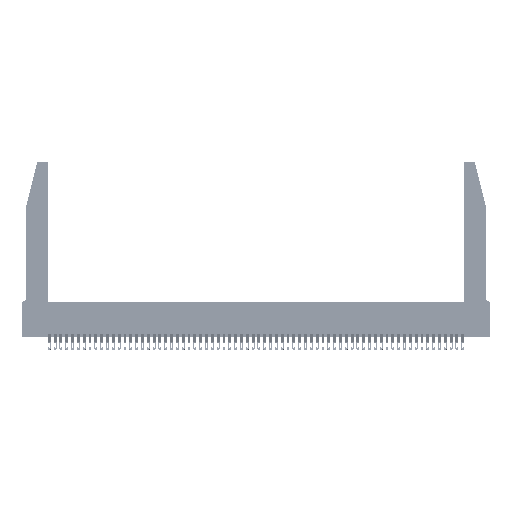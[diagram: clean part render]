
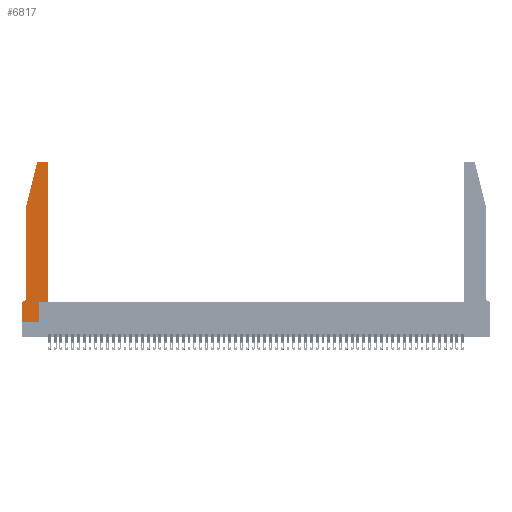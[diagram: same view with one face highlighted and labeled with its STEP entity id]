
A CAD part, top view. The second image highlights one B-rep face of the part: STEP entity #6817.
In plain terms, the highlighted planar face has unit normal (0, 0, 1).
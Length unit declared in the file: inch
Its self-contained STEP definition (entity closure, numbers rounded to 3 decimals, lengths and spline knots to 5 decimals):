
#1048 = VERTEX_POINT ( 'NONE', #35575 ) ;
#1233 = VERTEX_POINT ( 'NONE', #45393 ) ;
#1956 = DIRECTION ( 'NONE',  ( 0., 1., 0. ) ) ;
#2176 = CARTESIAN_POINT ( 'NONE',  ( 0.284, 2.75, 0.37 ) ) ;
#3952 = LINE ( 'NONE', #24320, #27723 ) ;
#5783 = AXIS2_PLACEMENT_3D ( 'NONE', #39515, #8673, #39702 ) ;
#5968 = LINE ( 'NONE', #25566, #29686 ) ;
#6336 = DIRECTION ( 'NONE',  ( 0., 0., 1. ) ) ;
#6624 = DIRECTION ( 'NONE',  ( -0.239, -0.971, 0. ) ) ;
#6817 = ADVANCED_FACE ( 'NONE', ( #33109 ), #57195, .T. ) ;
#8673 = DIRECTION ( 'NONE',  ( 0., 0., 1. ) ) ;
#8991 = LINE ( 'NONE', #37666, #54625 ) ;
#9388 = VECTOR ( 'NONE', #22037, 39.37008 ) ;
#9606 = ORIENTED_EDGE ( 'NONE', *, *, #15689, .T. ) ;
#9902 = VECTOR ( 'NONE', #38142, 39.37008 ) ;
#10875 = CARTESIAN_POINT ( 'NONE',  ( 0.0055, 0.35, 0.37 ) ) ;
#11460 = VERTEX_POINT ( 'NONE', #50817 ) ;
#11614 = CARTESIAN_POINT ( 'NONE',  ( 0.0755, 0.35, 0.37 ) ) ;
#11768 = CARTESIAN_POINT ( 'NONE',  ( 0.2605, 2.75, 0.37 ) ) ;
#12643 = CARTESIAN_POINT ( 'NONE',  ( 0.0755, 2., 0.37 ) ) ;
#13379 = EDGE_CURVE ( 'NONE', #26107, #41893, #55139, .T. ) ;
#13888 = DIRECTION ( 'NONE',  ( 0., 0., -1. ) ) ;
#14454 = DIRECTION ( 'NONE',  ( 1., 0., 0. ) ) ;
#15689 = EDGE_CURVE ( 'NONE', #21227, #52865, #30096, .T. ) ;
#15892 = CARTESIAN_POINT ( 'NONE',  ( 0.4505, 0.35, 0.37 ) ) ;
#17640 = EDGE_CURVE ( 'NONE', #41893, #39931, #25126, .T. ) ;
#17694 = CARTESIAN_POINT ( 'NONE',  ( 0.4505, 2.72, 0.37 ) ) ;
#17924 = ORIENTED_EDGE ( 'NONE', *, *, #28696, .T. ) ;
#19834 = DIRECTION ( 'NONE',  ( 0., -1., 0. ) ) ;
#20935 = ORIENTED_EDGE ( 'NONE', *, *, #45521, .T. ) ;
#21110 = VECTOR ( 'NONE', #42333, 39.37008 ) ;
#21181 = EDGE_LOOP ( 'NONE', ( #31744, #45854, #48638, #26102, #39755, #17924, #37886, #22853, #50915, #9606, #20935, #30724 ) ) ;
#21227 = VERTEX_POINT ( 'NONE', #34133 ) ;
#21753 = VECTOR ( 'NONE', #14454, 39.37008 ) ;
#21771 = EDGE_CURVE ( 'NONE', #11460, #1233, #30501, .T. ) ;
#22037 = DIRECTION ( 'NONE',  ( 0., -1., 0. ) ) ;
#22853 = ORIENTED_EDGE ( 'NONE', *, *, #29841, .T. ) ;
#23035 = VERTEX_POINT ( 'NONE', #49977 ) ;
#24320 = CARTESIAN_POINT ( 'NONE',  ( 0.4505, 0.35, 0.37 ) ) ;
#25126 = LINE ( 'NONE', #11768, #47162 ) ;
#25566 = CARTESIAN_POINT ( 'NONE',  ( 0.2865, 0.35, 0.37 ) ) ;
#26102 = ORIENTED_EDGE ( 'NONE', *, *, #42022, .T. ) ;
#26107 = VERTEX_POINT ( 'NONE', #17694 ) ;
#26424 = DIRECTION ( 'NONE',  ( 0., 0., 1. ) ) ;
#27723 = VECTOR ( 'NONE', #1956, 39.37008 ) ;
#28696 = EDGE_CURVE ( 'NONE', #52550, #11460, #56933, .T. ) ;
#29686 = VECTOR ( 'NONE', #51931, 39.37008 ) ;
#29841 = EDGE_CURVE ( 'NONE', #1233, #23035, #34834, .T. ) ;
#30096 = LINE ( 'NONE', #15892, #21110 ) ;
#30501 = LINE ( 'NONE', #46244, #55295 ) ;
#30724 = ORIENTED_EDGE ( 'NONE', *, *, #13379, .T. ) ;
#31416 = CARTESIAN_POINT ( 'NONE',  ( 0.4505, 0.35, 0.37 ) ) ;
#31744 = ORIENTED_EDGE ( 'NONE', *, *, #17640, .T. ) ;
#32039 = EDGE_CURVE ( 'NONE', #39931, #1048, #54001, .T. ) ;
#32960 = CARTESIAN_POINT ( 'NONE',  ( 0.284, 2.72, 0.37 ) ) ;
#33109 = FACE_OUTER_BOUND ( 'NONE', #21181, .T. ) ;
#33179 = EDGE_CURVE ( 'NONE', #53148, #52550, #34674, .T. ) ;
#34133 = CARTESIAN_POINT ( 'NONE',  ( 0.2865, 0.35, 0.37 ) ) ;
#34674 = CIRCLE ( 'NONE', #55115, 0.07 ) ;
#34817 = EDGE_CURVE ( 'NONE', #23035, #21227, #5968, .T. ) ;
#34834 = LINE ( 'NONE', #49765, #21753 ) ;
#35575 = CARTESIAN_POINT ( 'NONE',  ( 0.25487, 2.72718, 0.37 ) ) ;
#37367 = DIRECTION ( 'NONE',  ( 1., 0., 0. ) ) ;
#37666 = CARTESIAN_POINT ( 'NONE',  ( 0.0755, 2., 0.37 ) ) ;
#37886 = ORIENTED_EDGE ( 'NONE', *, *, #21771, .T. ) ;
#38142 = DIRECTION ( 'NONE',  ( -1., 0., 0. ) ) ;
#38417 = VERTEX_POINT ( 'NONE', #12643 ) ;
#39515 = CARTESIAN_POINT ( 'NONE',  ( 0., 0.35, 0.37 ) ) ;
#39565 = EDGE_CURVE ( 'NONE', #1048, #38417, #8991, .T. ) ;
#39702 = DIRECTION ( 'NONE',  ( 1., 0., 0. ) ) ;
#39755 = ORIENTED_EDGE ( 'NONE', *, *, #33179, .T. ) ;
#39931 = VERTEX_POINT ( 'NONE', #2176 ) ;
#40370 = CARTESIAN_POINT ( 'NONE',  ( 0.0055, 0.42, 0.37 ) ) ;
#41893 = VERTEX_POINT ( 'NONE', #56303 ) ;
#42022 = EDGE_CURVE ( 'NONE', #38417, #53148, #43368, .T. ) ;
#42333 = DIRECTION ( 'NONE',  ( 1., 0., 0. ) ) ;
#42730 = DIRECTION ( 'NONE',  ( -1., 0., 0. ) ) ;
#43368 = LINE ( 'NONE', #48417, #9388 ) ;
#43688 = AXIS2_PLACEMENT_3D ( 'NONE', #32960, #6336, #37367 ) ;
#44804 = DIRECTION ( 'NONE',  ( -1., 0., 0. ) ) ;
#45393 = CARTESIAN_POINT ( 'NONE',  ( 0., 0., 0.37 ) ) ;
#45521 = EDGE_CURVE ( 'NONE', #52865, #26107, #3952, .T. ) ;
#45854 = ORIENTED_EDGE ( 'NONE', *, *, #32039, .T. ) ;
#46131 = AXIS2_PLACEMENT_3D ( 'NONE', #52781, #26424, #57212 ) ;
#46244 = CARTESIAN_POINT ( 'NONE',  ( 0., 0., 0.37 ) ) ;
#47162 = VECTOR ( 'NONE', #42730, 39.37008 ) ;
#48417 = CARTESIAN_POINT ( 'NONE',  ( 0.0755, 2., 0.37 ) ) ;
#48638 = ORIENTED_EDGE ( 'NONE', *, *, #39565, .T. ) ;
#49765 = CARTESIAN_POINT ( 'NONE',  ( 0., 0., 0.37 ) ) ;
#49977 = CARTESIAN_POINT ( 'NONE',  ( 0.2865, 0., 0.37 ) ) ;
#50817 = CARTESIAN_POINT ( 'NONE',  ( 0., 0.35, 0.37 ) ) ;
#50915 = ORIENTED_EDGE ( 'NONE', *, *, #34817, .T. ) ;
#51931 = DIRECTION ( 'NONE',  ( 0., 1., 0. ) ) ;
#52550 = VERTEX_POINT ( 'NONE', #10875 ) ;
#52781 = CARTESIAN_POINT ( 'NONE',  ( 0.4205, 2.72, 0.37 ) ) ;
#52865 = VERTEX_POINT ( 'NONE', #31416 ) ;
#53148 = VERTEX_POINT ( 'NONE', #55430 ) ;
#54001 = CIRCLE ( 'NONE', #43688, 0.03 ) ;
#54625 = VECTOR ( 'NONE', #6624, 39.37008 ) ;
#55115 = AXIS2_PLACEMENT_3D ( 'NONE', #40370, #13888, #44804 ) ;
#55139 = CIRCLE ( 'NONE', #46131, 0.03 ) ;
#55295 = VECTOR ( 'NONE', #19834, 39.37008 ) ;
#55430 = CARTESIAN_POINT ( 'NONE',  ( 0.0755, 0.42, 0.37 ) ) ;
#56303 = CARTESIAN_POINT ( 'NONE',  ( 0.4205, 2.75, 0.37 ) ) ;
#56933 = LINE ( 'NONE', #11614, #9902 ) ;
#57195 = PLANE ( 'NONE',  #5783 ) ;
#57212 = DIRECTION ( 'NONE',  ( 1., 0., 0. ) ) ;
